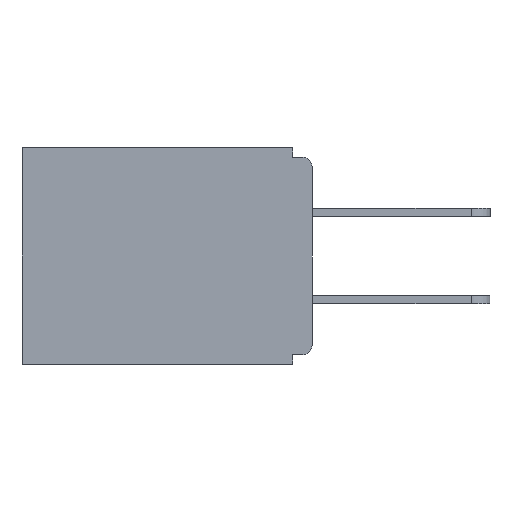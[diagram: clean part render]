
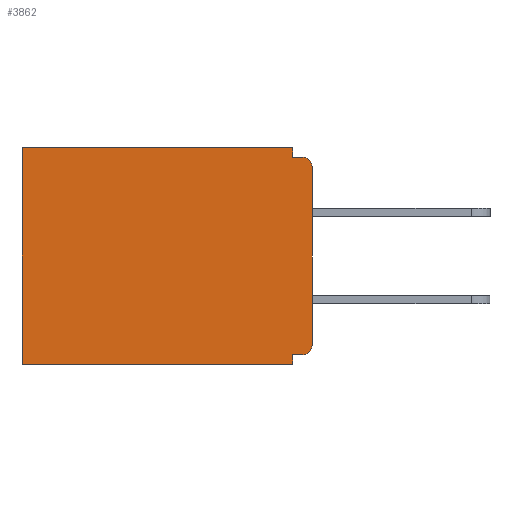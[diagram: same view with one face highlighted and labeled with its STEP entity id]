
A CAD part, left-side view. The second image highlights one B-rep face of the part: STEP entity #3862.
In plain terms, the highlighted planar face has unit normal (-1, 0, 0).
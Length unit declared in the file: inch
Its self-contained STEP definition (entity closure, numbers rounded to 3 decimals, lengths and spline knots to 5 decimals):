
#95 = VECTOR ( 'NONE', #4347, 39.37008 ) ;
#138 = ORIENTED_EDGE ( 'NONE', *, *, #1435, .F. ) ;
#499 = VECTOR ( 'NONE', #11140, 39.37008 ) ;
#558 = VECTOR ( 'NONE', #7734, 39.37008 ) ;
#672 = DIRECTION ( 'NONE',  ( 0., 0., -1. ) ) ;
#866 = PLANE ( 'NONE',  #2840 ) ;
#977 = LINE ( 'NONE', #7291, #499 ) ;
#1047 = VECTOR ( 'NONE', #6240, 39.37008 ) ;
#1435 = EDGE_CURVE ( 'NONE', #3697, #8741, #11659, .T. ) ;
#1498 = CARTESIAN_POINT ( 'NONE',  ( 0.298, 0., -0.015 ) ) ;
#1730 = EDGE_CURVE ( 'NONE', #9867, #12007, #8616, .T. ) ;
#1838 = LINE ( 'NONE', #8221, #1047 ) ;
#1932 = CARTESIAN_POINT ( 'NONE',  ( 0.298, 0., 0. ) ) ;
#1967 = DIRECTION ( 'NONE',  ( 0., 0., -1. ) ) ;
#2010 = LINE ( 'NONE', #5400, #9285 ) ;
#2542 = ORIENTED_EDGE ( 'NONE', *, *, #1730, .F. ) ;
#2627 = VERTEX_POINT ( 'NONE', #11848 ) ;
#2840 = AXIS2_PLACEMENT_3D ( 'NONE', #1932, #5812, #1967 ) ;
#3117 = EDGE_CURVE ( 'NONE', #11840, #9867, #7978, .T. ) ;
#3146 = ORIENTED_EDGE ( 'NONE', *, *, #5797, .F. ) ;
#3357 = DIRECTION ( 'NONE',  ( 0., -1., 0. ) ) ;
#3382 = DIRECTION ( 'NONE',  ( -1., 0., 0. ) ) ;
#3401 = CARTESIAN_POINT ( 'NONE',  ( 0.298, 0.031, -0.015 ) ) ;
#3415 = CARTESIAN_POINT ( 'NONE',  ( 0.298, 0., -0.313 ) ) ;
#3697 = VERTEX_POINT ( 'NONE', #3401 ) ;
#3737 = CARTESIAN_POINT ( 'NONE',  ( 0.298, 0., -0.03 ) ) ;
#3780 = CARTESIAN_POINT ( 'NONE',  ( 0.298, 0.015, -0.03 ) ) ;
#3862 = ADVANCED_FACE ( 'NONE', ( #11732 ), #866, .F. ) ;
#4321 = ORIENTED_EDGE ( 'NONE', *, *, #6786, .T. ) ;
#4347 = DIRECTION ( 'NONE',  ( 0., 0., -1. ) ) ;
#4747 = EDGE_CURVE ( 'NONE', #2627, #3697, #4807, .T. ) ;
#4807 = LINE ( 'NONE', #6226, #95 ) ;
#5329 = DIRECTION ( 'NONE',  ( 0., 1., 0. ) ) ;
#5400 = CARTESIAN_POINT ( 'NONE',  ( 0.298, 0., 0. ) ) ;
#5404 = CARTESIAN_POINT ( 'NONE',  ( 0.298, 0.015, -0.313 ) ) ;
#5532 = DIRECTION ( 'NONE',  ( -1., 0., 0. ) ) ;
#5635 = DIRECTION ( 'NONE',  ( 0., 0., -1. ) ) ;
#5671 = CARTESIAN_POINT ( 'NONE',  ( 0.298, 0.031, -0.343 ) ) ;
#5783 = CIRCLE ( 'NONE', #8471, 0.015 ) ;
#5797 = EDGE_CURVE ( 'NONE', #6926, #10897, #8396, .T. ) ;
#5812 = DIRECTION ( 'NONE',  ( 1., 0., 0. ) ) ;
#5880 = CARTESIAN_POINT ( 'NONE',  ( 0.298, 0.031, -0.328 ) ) ;
#6226 = CARTESIAN_POINT ( 'NONE',  ( 0.298, 0.031, -0.343 ) ) ;
#6240 = DIRECTION ( 'NONE',  ( 0., 1., 0. ) ) ;
#6786 = EDGE_CURVE ( 'NONE', #2627, #7722, #2010, .T. ) ;
#6879 = CARTESIAN_POINT ( 'NONE',  ( 0.298, 0.015, -0.015 ) ) ;
#6926 = VERTEX_POINT ( 'NONE', #3737 ) ;
#7050 = CIRCLE ( 'NONE', #11024, 0.015 ) ;
#7268 = EDGE_CURVE ( 'NONE', #11840, #10897, #5783, .T. ) ;
#7291 = CARTESIAN_POINT ( 'NONE',  ( 0.298, 0.46, 0. ) ) ;
#7377 = CARTESIAN_POINT ( 'NONE',  ( 0.298, 0.031, -0.343 ) ) ;
#7722 = VERTEX_POINT ( 'NONE', #9422 ) ;
#7734 = DIRECTION ( 'NONE',  ( 0., 0., -1. ) ) ;
#7797 = EDGE_CURVE ( 'NONE', #12007, #11803, #1838, .T. ) ;
#7975 = ORIENTED_EDGE ( 'NONE', *, *, #11505, .T. ) ;
#7978 = LINE ( 'NONE', #12018, #9357 ) ;
#7984 = ORIENTED_EDGE ( 'NONE', *, *, #11411, .T. ) ;
#8053 = ORIENTED_EDGE ( 'NONE', *, *, #3117, .F. ) ;
#8221 = CARTESIAN_POINT ( 'NONE',  ( 0.298, 0., -0.343 ) ) ;
#8256 = DIRECTION ( 'NONE',  ( 0., 0., -1. ) ) ;
#8396 = LINE ( 'NONE', #9492, #12302 ) ;
#8471 = AXIS2_PLACEMENT_3D ( 'NONE', #5404, #3382, #8256 ) ;
#8616 = LINE ( 'NONE', #5671, #558 ) ;
#8741 = VERTEX_POINT ( 'NONE', #6879 ) ;
#9105 = CARTESIAN_POINT ( 'NONE',  ( 0.298, 0.46, -0.343 ) ) ;
#9285 = VECTOR ( 'NONE', #12170, 39.37008 ) ;
#9357 = VECTOR ( 'NONE', #5329, 39.37008 ) ;
#9422 = CARTESIAN_POINT ( 'NONE',  ( 0.298, 0.46, 0. ) ) ;
#9492 = CARTESIAN_POINT ( 'NONE',  ( 0.298, 0., 0. ) ) ;
#9867 = VERTEX_POINT ( 'NONE', #5880 ) ;
#10186 = CARTESIAN_POINT ( 'NONE',  ( 0.298, 0.015, -0.328 ) ) ;
#10562 = ORIENTED_EDGE ( 'NONE', *, *, #4747, .F. ) ;
#10897 = VERTEX_POINT ( 'NONE', #3415 ) ;
#10914 = VECTOR ( 'NONE', #3357, 39.37008 ) ;
#11024 = AXIS2_PLACEMENT_3D ( 'NONE', #3780, #5532, #672 ) ;
#11140 = DIRECTION ( 'NONE',  ( 0., 0., -1. ) ) ;
#11341 = ORIENTED_EDGE ( 'NONE', *, *, #7268, .T. ) ;
#11411 = EDGE_CURVE ( 'NONE', #7722, #11803, #977, .T. ) ;
#11505 = EDGE_CURVE ( 'NONE', #6926, #8741, #7050, .T. ) ;
#11507 = ORIENTED_EDGE ( 'NONE', *, *, #7797, .F. ) ;
#11659 = LINE ( 'NONE', #1498, #10914 ) ;
#11732 = FACE_OUTER_BOUND ( 'NONE', #12026, .T. ) ;
#11803 = VERTEX_POINT ( 'NONE', #9105 ) ;
#11840 = VERTEX_POINT ( 'NONE', #10186 ) ;
#11848 = CARTESIAN_POINT ( 'NONE',  ( 0.298, 0.031, 0. ) ) ;
#12007 = VERTEX_POINT ( 'NONE', #7377 ) ;
#12018 = CARTESIAN_POINT ( 'NONE',  ( 0.298, 0., -0.328 ) ) ;
#12026 = EDGE_LOOP ( 'NONE', ( #7975, #138, #10562, #4321, #7984, #11507, #2542, #8053, #11341, #3146 ) ) ;
#12170 = DIRECTION ( 'NONE',  ( 0., 1., 0. ) ) ;
#12302 = VECTOR ( 'NONE', #5635, 39.37008 ) ;
